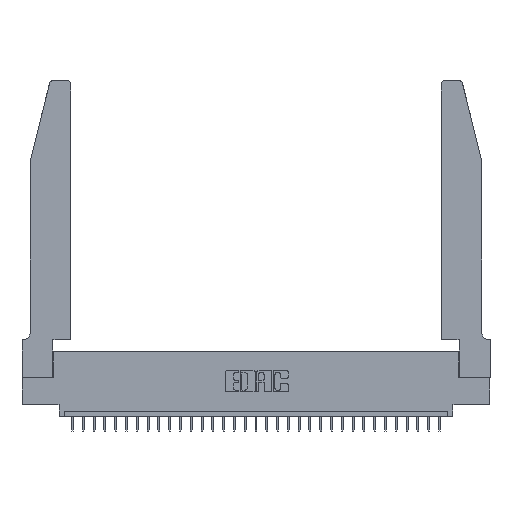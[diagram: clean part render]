
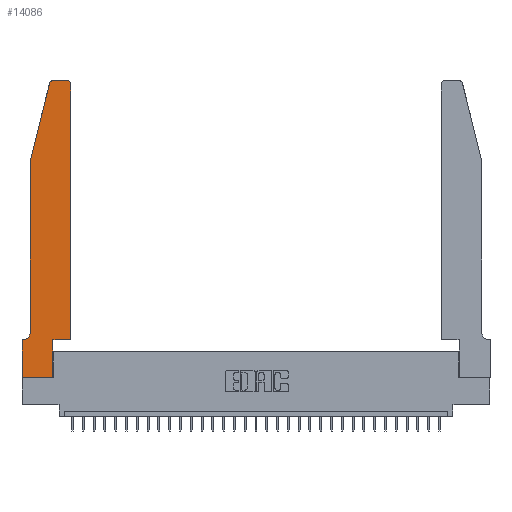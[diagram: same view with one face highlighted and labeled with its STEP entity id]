
A CAD part, top view. The second image highlights one B-rep face of the part: STEP entity #14086.
In plain terms, the highlighted planar face has unit normal (0, 0, 1).
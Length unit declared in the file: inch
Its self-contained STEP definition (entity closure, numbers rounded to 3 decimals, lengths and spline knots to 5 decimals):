
#260 = ORIENTED_EDGE ( 'NONE', *, *, #32005, .T. ) ;
#753 = LINE ( 'NONE', #5811, #1936 ) ;
#1462 = CARTESIAN_POINT ( 'NONE',  ( 0., 0., 0.37 ) ) ;
#1887 = VECTOR ( 'NONE', #25180, 39.37008 ) ;
#1936 = VECTOR ( 'NONE', #13482, 39.37008 ) ;
#2505 = CARTESIAN_POINT ( 'NONE',  ( 0.2605, 2.75, 0.37 ) ) ;
#2895 = ORIENTED_EDGE ( 'NONE', *, *, #19952, .T. ) ;
#2899 = CIRCLE ( 'NONE', #14887, 0.03 ) ;
#2928 = CIRCLE ( 'NONE', #13363, 0.03 ) ;
#4171 = VERTEX_POINT ( 'NONE', #6273 ) ;
#4603 = LINE ( 'NONE', #32176, #4680 ) ;
#4680 = VECTOR ( 'NONE', #18973, 39.37008 ) ;
#4828 = CARTESIAN_POINT ( 'NONE',  ( 0.0755, 2., 0.37 ) ) ;
#5586 = EDGE_CURVE ( 'NONE', #25420, #27899, #30685, .T. ) ;
#5714 = DIRECTION ( 'NONE',  ( 1., 0., 0. ) ) ;
#5811 = CARTESIAN_POINT ( 'NONE',  ( 0.4505, 0.35, 0.37 ) ) ;
#6167 = CARTESIAN_POINT ( 'NONE',  ( 0., 0., 0.37 ) ) ;
#6273 = CARTESIAN_POINT ( 'NONE',  ( 0.0055, 0.35, 0.37 ) ) ;
#6767 = EDGE_CURVE ( 'NONE', #28661, #25420, #13394, .T. ) ;
#7040 = CARTESIAN_POINT ( 'NONE',  ( 0.2865, 0.35, 0.37 ) ) ;
#7348 = LINE ( 'NONE', #12241, #21103 ) ;
#7436 = DIRECTION ( 'NONE',  ( -0.239, -0.971, 0. ) ) ;
#7464 = EDGE_CURVE ( 'NONE', #7980, #22272, #22601, .T. ) ;
#7766 = VECTOR ( 'NONE', #5714, 39.37008 ) ;
#7922 = ORIENTED_EDGE ( 'NONE', *, *, #18785, .T. ) ;
#7980 = VERTEX_POINT ( 'NONE', #13116 ) ;
#8120 = CARTESIAN_POINT ( 'NONE',  ( 0., 0.35, 0.37 ) ) ;
#8304 = ORIENTED_EDGE ( 'NONE', *, *, #21125, .T. ) ;
#8457 = VERTEX_POINT ( 'NONE', #30060 ) ;
#8973 = AXIS2_PLACEMENT_3D ( 'NONE', #12534, #29665, #9779 ) ;
#9458 = VECTOR ( 'NONE', #7436, 39.37008 ) ;
#9732 = EDGE_CURVE ( 'NONE', #10705, #7980, #31919, .T. ) ;
#9779 = DIRECTION ( 'NONE',  ( -1., 0., 0. ) ) ;
#10572 = EDGE_CURVE ( 'NONE', #22272, #4171, #17302, .T. ) ;
#10705 = VERTEX_POINT ( 'NONE', #20843 ) ;
#10784 = DIRECTION ( 'NONE',  ( 0., -1., 0. ) ) ;
#11224 = DIRECTION ( 'NONE',  ( 0., 0., 1. ) ) ;
#12024 = CARTESIAN_POINT ( 'NONE',  ( 0.2865, 0., 0.37 ) ) ;
#12241 = CARTESIAN_POINT ( 'NONE',  ( 0.4505, 0.35, 0.37 ) ) ;
#12472 = VECTOR ( 'NONE', #22767, 39.37008 ) ;
#12534 = CARTESIAN_POINT ( 'NONE',  ( 0.0055, 0.42, 0.37 ) ) ;
#12578 = DIRECTION ( 'NONE',  ( 0., 1., 0. ) ) ;
#12791 = LINE ( 'NONE', #7040, #17010 ) ;
#13116 = CARTESIAN_POINT ( 'NONE',  ( 0.0755, 2., 0.37 ) ) ;
#13301 = ORIENTED_EDGE ( 'NONE', *, *, #21070, .T. ) ;
#13362 = CARTESIAN_POINT ( 'NONE',  ( 0.2865, 0.35, 0.37 ) ) ;
#13363 = AXIS2_PLACEMENT_3D ( 'NONE', #15524, #14437, #24720 ) ;
#13394 = LINE ( 'NONE', #1462, #14091 ) ;
#13482 = DIRECTION ( 'NONE',  ( 0., 1., 0. ) ) ;
#13836 = CARTESIAN_POINT ( 'NONE',  ( 0., 0.35, 0.37 ) ) ;
#14086 = ADVANCED_FACE ( 'NONE', ( #18255 ), #23623, .T. ) ;
#14091 = VECTOR ( 'NONE', #10784, 39.37008 ) ;
#14403 = ORIENTED_EDGE ( 'NONE', *, *, #7464, .T. ) ;
#14437 = DIRECTION ( 'NONE',  ( 0., 0., 1. ) ) ;
#14791 = ORIENTED_EDGE ( 'NONE', *, *, #10572, .T. ) ;
#14887 = AXIS2_PLACEMENT_3D ( 'NONE', #16077, #20978, #30937 ) ;
#15223 = LINE ( 'NONE', #2505, #1887 ) ;
#15401 = VERTEX_POINT ( 'NONE', #15966 ) ;
#15524 = CARTESIAN_POINT ( 'NONE',  ( 0.4205, 2.72, 0.37 ) ) ;
#15966 = CARTESIAN_POINT ( 'NONE',  ( 0.4505, 2.72, 0.37 ) ) ;
#16077 = CARTESIAN_POINT ( 'NONE',  ( 0.284, 2.72, 0.37 ) ) ;
#16925 = ORIENTED_EDGE ( 'NONE', *, *, #6767, .T. ) ;
#16961 = VERTEX_POINT ( 'NONE', #31056 ) ;
#17010 = VECTOR ( 'NONE', #12578, 39.37008 ) ;
#17256 = ORIENTED_EDGE ( 'NONE', *, *, #20139, .T. ) ;
#17302 = CIRCLE ( 'NONE', #8973, 0.07 ) ;
#18255 = FACE_OUTER_BOUND ( 'NONE', #23101, .T. ) ;
#18757 = CARTESIAN_POINT ( 'NONE',  ( 0., 0., 0.37 ) ) ;
#18785 = EDGE_CURVE ( 'NONE', #25304, #8457, #7348, .T. ) ;
#18893 = DIRECTION ( 'NONE',  ( 1., 0., 0. ) ) ;
#18973 = DIRECTION ( 'NONE',  ( -1., 0., 0. ) ) ;
#19952 = EDGE_CURVE ( 'NONE', #27899, #25304, #12791, .T. ) ;
#20139 = EDGE_CURVE ( 'NONE', #16961, #21712, #15223, .T. ) ;
#20843 = CARTESIAN_POINT ( 'NONE',  ( 0.25487, 2.72718, 0.37 ) ) ;
#20978 = DIRECTION ( 'NONE',  ( 0., 0., 1. ) ) ;
#21070 = EDGE_CURVE ( 'NONE', #8457, #15401, #753, .T. ) ;
#21103 = VECTOR ( 'NONE', #29851, 39.37008 ) ;
#21125 = EDGE_CURVE ( 'NONE', #21712, #10705, #2899, .T. ) ;
#21712 = VERTEX_POINT ( 'NONE', #30209 ) ;
#22272 = VERTEX_POINT ( 'NONE', #25765 ) ;
#22601 = LINE ( 'NONE', #30109, #12472 ) ;
#22767 = DIRECTION ( 'NONE',  ( 0., -1., 0. ) ) ;
#23101 = EDGE_LOOP ( 'NONE', ( #17256, #8304, #31068, #14403, #14791, #25116, #16925, #30113, #2895, #7922, #13301, #260 ) ) ;
#23623 = PLANE ( 'NONE',  #25727 ) ;
#24720 = DIRECTION ( 'NONE',  ( 1., 0., 0. ) ) ;
#25116 = ORIENTED_EDGE ( 'NONE', *, *, #26010, .T. ) ;
#25180 = DIRECTION ( 'NONE',  ( -1., 0., 0. ) ) ;
#25304 = VERTEX_POINT ( 'NONE', #13362 ) ;
#25420 = VERTEX_POINT ( 'NONE', #6167 ) ;
#25727 = AXIS2_PLACEMENT_3D ( 'NONE', #13836, #11224, #18893 ) ;
#25765 = CARTESIAN_POINT ( 'NONE',  ( 0.0755, 0.42, 0.37 ) ) ;
#26010 = EDGE_CURVE ( 'NONE', #4171, #28661, #4603, .T. ) ;
#27899 = VERTEX_POINT ( 'NONE', #12024 ) ;
#28661 = VERTEX_POINT ( 'NONE', #8120 ) ;
#29665 = DIRECTION ( 'NONE',  ( 0., 0., -1. ) ) ;
#29851 = DIRECTION ( 'NONE',  ( 1., 0., 0. ) ) ;
#30060 = CARTESIAN_POINT ( 'NONE',  ( 0.4505, 0.35, 0.37 ) ) ;
#30109 = CARTESIAN_POINT ( 'NONE',  ( 0.0755, 2., 0.37 ) ) ;
#30113 = ORIENTED_EDGE ( 'NONE', *, *, #5586, .T. ) ;
#30209 = CARTESIAN_POINT ( 'NONE',  ( 0.284, 2.75, 0.37 ) ) ;
#30685 = LINE ( 'NONE', #18757, #7766 ) ;
#30937 = DIRECTION ( 'NONE',  ( 1., 0., 0. ) ) ;
#31056 = CARTESIAN_POINT ( 'NONE',  ( 0.4205, 2.75, 0.37 ) ) ;
#31068 = ORIENTED_EDGE ( 'NONE', *, *, #9732, .T. ) ;
#31919 = LINE ( 'NONE', #4828, #9458 ) ;
#32005 = EDGE_CURVE ( 'NONE', #15401, #16961, #2928, .T. ) ;
#32176 = CARTESIAN_POINT ( 'NONE',  ( 0.0755, 0.35, 0.37 ) ) ;
